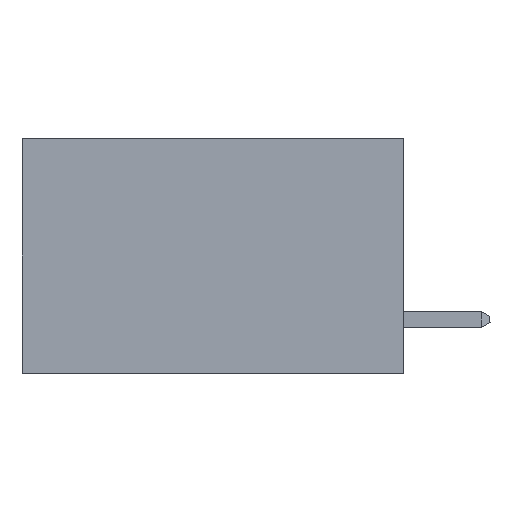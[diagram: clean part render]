
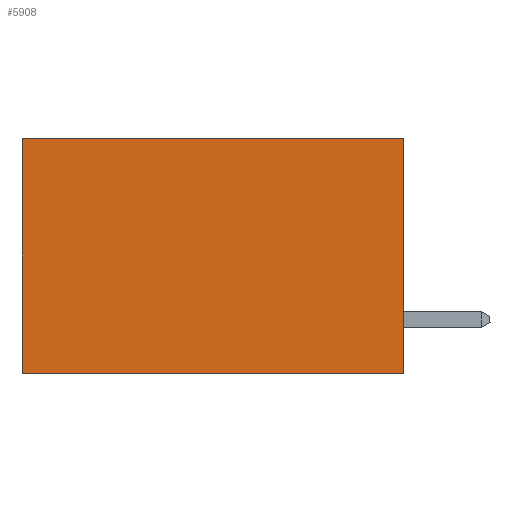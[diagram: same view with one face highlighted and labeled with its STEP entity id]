
A CAD part, left-side view. The second image highlights one B-rep face of the part: STEP entity #5908.
In plain terms, the highlighted planar face has unit normal (-1, 0, 0).
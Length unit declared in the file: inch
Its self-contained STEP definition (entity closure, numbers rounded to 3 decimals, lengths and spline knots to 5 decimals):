
#233 = CARTESIAN_POINT ( 'NONE',  ( 0.2875, 0., -0.37 ) ) ;
#568 = VECTOR ( 'NONE', #6481, 39.37008 ) ;
#1587 = VERTEX_POINT ( 'NONE', #15877 ) ;
#1680 = VERTEX_POINT ( 'NONE', #12299 ) ;
#1694 = FACE_OUTER_BOUND ( 'NONE', #8037, .T. ) ;
#2293 = ORIENTED_EDGE ( 'NONE', *, *, #25851, .F. ) ;
#4827 = VECTOR ( 'NONE', #26446, 39.37008 ) ;
#4832 = CARTESIAN_POINT ( 'NONE',  ( 0.2875, 0.6, 0. ) ) ;
#5191 = ORIENTED_EDGE ( 'NONE', *, *, #9210, .T. ) ;
#5372 = ORIENTED_EDGE ( 'NONE', *, *, #33593, .T. ) ;
#5908 = ADVANCED_FACE ( 'NONE', ( #1694 ), #6030, .F. ) ;
#6030 = PLANE ( 'NONE',  #32748 ) ;
#6481 = DIRECTION ( 'NONE',  ( 0., 0., -1. ) ) ;
#8037 = EDGE_LOOP ( 'NONE', ( #5191, #23878, #2293, #5372 ) ) ;
#9210 = EDGE_CURVE ( 'NONE', #23741, #1680, #29188, .T. ) ;
#12299 = CARTESIAN_POINT ( 'NONE',  ( 0.2875, 0.6, -0.37 ) ) ;
#12824 = CARTESIAN_POINT ( 'NONE',  ( 0.2875, 0., 0. ) ) ;
#13045 = DIRECTION ( 'NONE',  ( 0., 1., 0. ) ) ;
#14199 = VECTOR ( 'NONE', #13045, 39.37008 ) ;
#15877 = CARTESIAN_POINT ( 'NONE',  ( 0.2875, 0., -0.37 ) ) ;
#17323 = LINE ( 'NONE', #18883, #31950 ) ;
#17991 = LINE ( 'NONE', #233, #4827 ) ;
#18883 = CARTESIAN_POINT ( 'NONE',  ( 0.2875, 0., 0. ) ) ;
#18990 = DIRECTION ( 'NONE',  ( 1., 0., 0. ) ) ;
#21413 = DIRECTION ( 'NONE',  ( 0., 0., -1. ) ) ;
#22372 = VERTEX_POINT ( 'NONE', #25814 ) ;
#23741 = VERTEX_POINT ( 'NONE', #33290 ) ;
#23878 = ORIENTED_EDGE ( 'NONE', *, *, #31877, .F. ) ;
#24368 = CARTESIAN_POINT ( 'NONE',  ( 0.2875, 0., 0. ) ) ;
#25814 = CARTESIAN_POINT ( 'NONE',  ( 0.2875, 0., 0. ) ) ;
#25851 = EDGE_CURVE ( 'NONE', #22372, #1587, #17323, .T. ) ;
#26446 = DIRECTION ( 'NONE',  ( 0., 1., 0. ) ) ;
#26985 = DIRECTION ( 'NONE',  ( 0., 0., -1. ) ) ;
#29188 = LINE ( 'NONE', #4832, #568 ) ;
#31877 = EDGE_CURVE ( 'NONE', #1587, #1680, #17991, .T. ) ;
#31950 = VECTOR ( 'NONE', #21413, 39.37008 ) ;
#32116 = LINE ( 'NONE', #12824, #14199 ) ;
#32748 = AXIS2_PLACEMENT_3D ( 'NONE', #24368, #18990, #26985 ) ;
#33290 = CARTESIAN_POINT ( 'NONE',  ( 0.2875, 0.6, 0. ) ) ;
#33593 = EDGE_CURVE ( 'NONE', #22372, #23741, #32116, .T. ) ;
